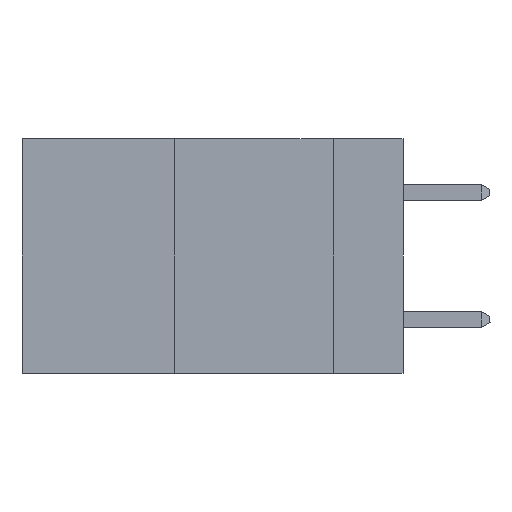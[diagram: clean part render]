
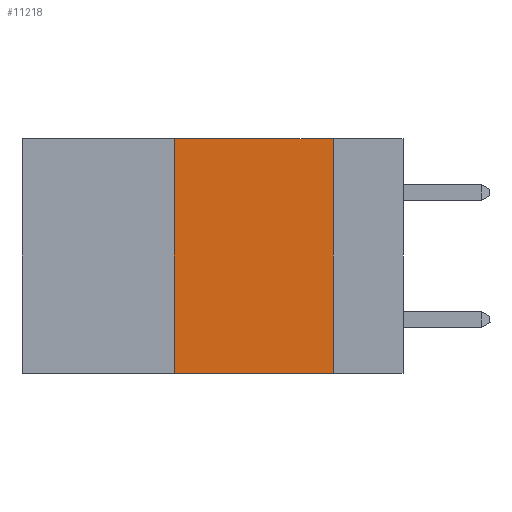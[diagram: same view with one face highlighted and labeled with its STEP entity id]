
A CAD part, left-side view. The second image highlights one B-rep face of the part: STEP entity #11218.
In plain terms, the highlighted planar face has unit normal (-1, 0, 0).
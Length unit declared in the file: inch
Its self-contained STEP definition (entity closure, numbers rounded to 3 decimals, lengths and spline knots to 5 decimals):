
#532 = EDGE_CURVE ( 'NONE', #32640, #20155, #12985, .T. ) ;
#1001 = PLANE ( 'NONE',  #25607 ) ;
#1596 = LINE ( 'NONE', #19418, #28294 ) ;
#2349 = VECTOR ( 'NONE', #7433, 39.37008 ) ;
#2560 = EDGE_CURVE ( 'NONE', #30721, #32886, #1596, .T. ) ;
#4987 = CARTESIAN_POINT ( 'NONE',  ( 0., 0.11, -0.37 ) ) ;
#6399 = CARTESIAN_POINT ( 'NONE',  ( 0., 0.36, 0. ) ) ;
#7106 = FACE_OUTER_BOUND ( 'NONE', #13156, .T. ) ;
#7433 = DIRECTION ( 'NONE',  ( 0., -1., 0. ) ) ;
#9825 = EDGE_CURVE ( 'NONE', #30721, #20155, #16586, .T. ) ;
#11133 = VECTOR ( 'NONE', #25125, 39.37008 ) ;
#11218 = ADVANCED_FACE ( 'NONE', ( #7106 ), #1001, .F. ) ;
#11947 = DIRECTION ( 'NONE',  ( 1., 0., 0. ) ) ;
#12652 = ORIENTED_EDGE ( 'NONE', *, *, #9825, .T. ) ;
#12985 = LINE ( 'NONE', #25787, #11133 ) ;
#13156 = EDGE_LOOP ( 'NONE', ( #25678, #24750, #26309, #12652 ) ) ;
#14283 = CARTESIAN_POINT ( 'NONE',  ( 0., 0.11, 0. ) ) ;
#16586 = LINE ( 'NONE', #29575, #27131 ) ;
#17460 = CARTESIAN_POINT ( 'NONE',  ( 0., 0.36, -0.37 ) ) ;
#19418 = CARTESIAN_POINT ( 'NONE',  ( 0., 0.36, 0. ) ) ;
#20155 = VERTEX_POINT ( 'NONE', #4987 ) ;
#20408 = LINE ( 'NONE', #30237, #2349 ) ;
#21758 = DIRECTION ( 'NONE',  ( 0., -1., 0. ) ) ;
#24750 = ORIENTED_EDGE ( 'NONE', *, *, #31443, .F. ) ;
#25125 = DIRECTION ( 'NONE',  ( 0., 0., -1. ) ) ;
#25607 = AXIS2_PLACEMENT_3D ( 'NONE', #29747, #11947, #27408 ) ;
#25678 = ORIENTED_EDGE ( 'NONE', *, *, #532, .F. ) ;
#25787 = CARTESIAN_POINT ( 'NONE',  ( 0., 0.11, 0. ) ) ;
#26309 = ORIENTED_EDGE ( 'NONE', *, *, #2560, .F. ) ;
#27131 = VECTOR ( 'NONE', #21758, 39.37008 ) ;
#27408 = DIRECTION ( 'NONE',  ( 0., 0., -1. ) ) ;
#28294 = VECTOR ( 'NONE', #29889, 39.37008 ) ;
#29575 = CARTESIAN_POINT ( 'NONE',  ( 0., 0.6, -0.37 ) ) ;
#29747 = CARTESIAN_POINT ( 'NONE',  ( 0., 0.6, 0. ) ) ;
#29889 = DIRECTION ( 'NONE',  ( 0., 0., 1. ) ) ;
#30237 = CARTESIAN_POINT ( 'NONE',  ( 0., 0.6, 0. ) ) ;
#30721 = VERTEX_POINT ( 'NONE', #17460 ) ;
#31443 = EDGE_CURVE ( 'NONE', #32886, #32640, #20408, .T. ) ;
#32640 = VERTEX_POINT ( 'NONE', #14283 ) ;
#32886 = VERTEX_POINT ( 'NONE', #6399 ) ;
